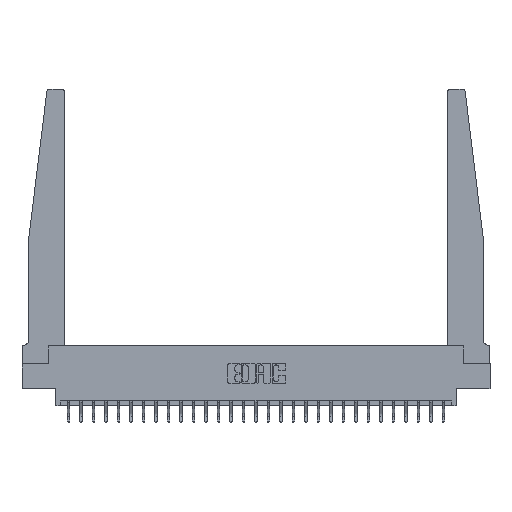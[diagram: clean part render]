
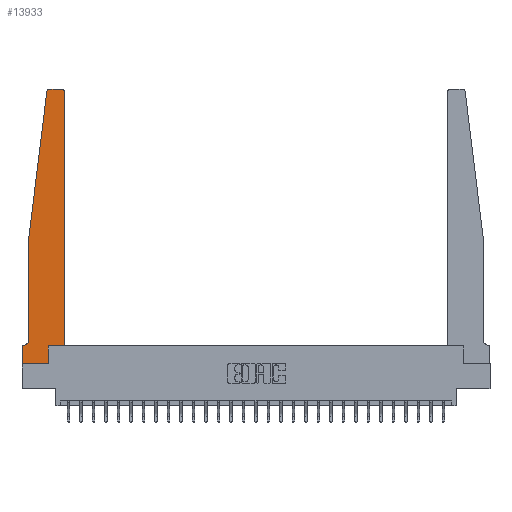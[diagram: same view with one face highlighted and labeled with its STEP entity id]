
A CAD part, top view. The second image highlights one B-rep face of the part: STEP entity #13933.
In plain terms, the highlighted planar face has unit normal (0, 0, 1).
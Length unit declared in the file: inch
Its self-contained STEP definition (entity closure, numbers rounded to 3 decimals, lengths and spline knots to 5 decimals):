
#178 = DIRECTION ( 'NONE',  ( 1., 0., 0. ) ) ;
#185 = DIRECTION ( 'NONE',  ( -1., 0., 0. ) ) ;
#621 = CARTESIAN_POINT ( 'NONE',  ( 0.425, 0.18, 0.37 ) ) ;
#720 = LINE ( 'NONE', #15102, #7549 ) ;
#905 = ORIENTED_EDGE ( 'NONE', *, *, #20341, .T. ) ;
#1428 = VERTEX_POINT ( 'NONE', #9687 ) ;
#1728 = FACE_OUTER_BOUND ( 'NONE', #15883, .T. ) ;
#1777 = VERTEX_POINT ( 'NONE', #15688 ) ;
#1837 = ORIENTED_EDGE ( 'NONE', *, *, #11413, .T. ) ;
#2087 = EDGE_CURVE ( 'NONE', #8320, #10356, #23120, .T. ) ;
#2580 = CARTESIAN_POINT ( 'NONE',  ( 0.015, 0.2375, 0.37 ) ) ;
#3020 = VECTOR ( 'NONE', #24836, 39.37008 ) ;
#3621 = EDGE_CURVE ( 'NONE', #24551, #7787, #3852, .T. ) ;
#3852 = LINE ( 'NONE', #12295, #3020 ) ;
#3930 = CARTESIAN_POINT ( 'NONE',  ( 0., 0.1875, 0.37 ) ) ;
#3963 = LINE ( 'NONE', #621, #8898 ) ;
#4074 = CARTESIAN_POINT ( 'NONE',  ( 0.24675, 2.72367, 0.37 ) ) ;
#4113 = EDGE_CURVE ( 'NONE', #1777, #4133, #22219, .T. ) ;
#4133 = VERTEX_POINT ( 'NONE', #25760 ) ;
#4425 = VERTEX_POINT ( 'NONE', #14247 ) ;
#4759 = AXIS2_PLACEMENT_3D ( 'NONE', #5615, #18304, #26724 ) ;
#5272 = CARTESIAN_POINT ( 'NONE',  ( 0.065, 1.25, 0.37 ) ) ;
#5615 = CARTESIAN_POINT ( 'NONE',  ( 0.395, 2.72, 0.37 ) ) ;
#6169 = CARTESIAN_POINT ( 'NONE',  ( 0.065, 0.1875, 0.37 ) ) ;
#6347 = LINE ( 'NONE', #21106, #18297 ) ;
#6387 = CIRCLE ( 'NONE', #25783, 0.03 ) ;
#6558 = CARTESIAN_POINT ( 'NONE',  ( 0., 0., 0.37 ) ) ;
#6650 = CARTESIAN_POINT ( 'NONE',  ( 0.27653, 2.72, 0.37 ) ) ;
#6946 = EDGE_CURVE ( 'NONE', #16618, #4425, #720, .T. ) ;
#7549 = VECTOR ( 'NONE', #23517, 39.37008 ) ;
#7787 = VERTEX_POINT ( 'NONE', #17882 ) ;
#8205 = AXIS2_PLACEMENT_3D ( 'NONE', #3930, #10163, #20774 ) ;
#8320 = VERTEX_POINT ( 'NONE', #8462 ) ;
#8462 = CARTESIAN_POINT ( 'NONE',  ( 0.395, 2.75, 0.37 ) ) ;
#8898 = VECTOR ( 'NONE', #26035, 39.37008 ) ;
#9370 = CARTESIAN_POINT ( 'NONE',  ( 0.425, 0.18, 0.37 ) ) ;
#9687 = CARTESIAN_POINT ( 'NONE',  ( 0.425, 2.72, 0.37 ) ) ;
#9797 = CARTESIAN_POINT ( 'NONE',  ( 0.27653, 2.75, 0.37 ) ) ;
#9954 = VERTEX_POINT ( 'NONE', #5272 ) ;
#10163 = DIRECTION ( 'NONE',  ( 0., 0., 1. ) ) ;
#10242 = CARTESIAN_POINT ( 'NONE',  ( 0.425, 0.18, 0.37 ) ) ;
#10336 = AXIS2_PLACEMENT_3D ( 'NONE', #2580, #23701, #19147 ) ;
#10356 = VERTEX_POINT ( 'NONE', #9797 ) ;
#11413 = EDGE_CURVE ( 'NONE', #10356, #15060, #6387, .T. ) ;
#11525 = LINE ( 'NONE', #26000, #15228 ) ;
#11565 = VECTOR ( 'NONE', #22717, 39.37008 ) ;
#11840 = EDGE_CURVE ( 'NONE', #15060, #9954, #6347, .T. ) ;
#12295 = CARTESIAN_POINT ( 'NONE',  ( 0., 0., 0.37 ) ) ;
#12315 = ORIENTED_EDGE ( 'NONE', *, *, #3621, .T. ) ;
#12587 = EDGE_CURVE ( 'NONE', #7787, #16618, #12894, .T. ) ;
#12894 = LINE ( 'NONE', #6558, #13046 ) ;
#13046 = VECTOR ( 'NONE', #178, 39.37008 ) ;
#13933 = ADVANCED_FACE ( 'NONE', ( #1728 ), #26854, .T. ) ;
#14226 = LINE ( 'NONE', #10242, #16449 ) ;
#14247 = CARTESIAN_POINT ( 'NONE',  ( 0.2605, 0.18, 0.37 ) ) ;
#14708 = CARTESIAN_POINT ( 'NONE',  ( 0.2605, 0., 0.37 ) ) ;
#15060 = VERTEX_POINT ( 'NONE', #4074 ) ;
#15102 = CARTESIAN_POINT ( 'NONE',  ( 0.2605, 0.18, 0.37 ) ) ;
#15228 = VECTOR ( 'NONE', #19922, 39.37008 ) ;
#15688 = CARTESIAN_POINT ( 'NONE',  ( 0.065, 0.2375, 0.37 ) ) ;
#15883 = EDGE_LOOP ( 'NONE', ( #23024, #1837, #20906, #24942, #17190, #905, #12315, #15890, #24903, #16985, #21485, #25228 ) ) ;
#15890 = ORIENTED_EDGE ( 'NONE', *, *, #12587, .T. ) ;
#16309 = DIRECTION ( 'NONE',  ( 0., 1., 0. ) ) ;
#16449 = VECTOR ( 'NONE', #16309, 39.37008 ) ;
#16460 = EDGE_CURVE ( 'NONE', #1428, #8320, #18410, .T. ) ;
#16618 = VERTEX_POINT ( 'NONE', #14708 ) ;
#16948 = VECTOR ( 'NONE', #185, 39.37008 ) ;
#16985 = ORIENTED_EDGE ( 'NONE', *, *, #20096, .T. ) ;
#17132 = DIRECTION ( 'NONE',  ( 1., 0., 0. ) ) ;
#17190 = ORIENTED_EDGE ( 'NONE', *, *, #4113, .T. ) ;
#17489 = VERTEX_POINT ( 'NONE', #9370 ) ;
#17882 = CARTESIAN_POINT ( 'NONE',  ( 0., 0., 0.37 ) ) ;
#18297 = VECTOR ( 'NONE', #25649, 39.37008 ) ;
#18304 = DIRECTION ( 'NONE',  ( 0., 0., 1. ) ) ;
#18410 = CIRCLE ( 'NONE', #4759, 0.03 ) ;
#18987 = LINE ( 'NONE', #6169, #11565 ) ;
#19147 = DIRECTION ( 'NONE',  ( -1., 0., 0. ) ) ;
#19922 = DIRECTION ( 'NONE',  ( 0., -1., 0. ) ) ;
#20096 = EDGE_CURVE ( 'NONE', #4425, #17489, #3963, .T. ) ;
#20341 = EDGE_CURVE ( 'NONE', #4133, #24551, #18987, .T. ) ;
#20774 = DIRECTION ( 'NONE',  ( 1., 0., 0. ) ) ;
#20906 = ORIENTED_EDGE ( 'NONE', *, *, #11840, .T. ) ;
#21106 = CARTESIAN_POINT ( 'NONE',  ( 0.065, 1.25, 0.37 ) ) ;
#21485 = ORIENTED_EDGE ( 'NONE', *, *, #22492, .T. ) ;
#22219 = CIRCLE ( 'NONE', #10336, 0.05 ) ;
#22492 = EDGE_CURVE ( 'NONE', #17489, #1428, #14226, .T. ) ;
#22717 = DIRECTION ( 'NONE',  ( -1., 0., 0. ) ) ;
#23024 = ORIENTED_EDGE ( 'NONE', *, *, #2087, .T. ) ;
#23120 = LINE ( 'NONE', #24922, #16948 ) ;
#23422 = CARTESIAN_POINT ( 'NONE',  ( 0., 0.1875, 0.37 ) ) ;
#23480 = DIRECTION ( 'NONE',  ( 0., 0., 1. ) ) ;
#23517 = DIRECTION ( 'NONE',  ( 0., 1., 0. ) ) ;
#23701 = DIRECTION ( 'NONE',  ( 0., 0., -1. ) ) ;
#24551 = VERTEX_POINT ( 'NONE', #23422 ) ;
#24836 = DIRECTION ( 'NONE',  ( 0., -1., 0. ) ) ;
#24903 = ORIENTED_EDGE ( 'NONE', *, *, #6946, .T. ) ;
#24922 = CARTESIAN_POINT ( 'NONE',  ( 0.25, 2.75, 0.37 ) ) ;
#24942 = ORIENTED_EDGE ( 'NONE', *, *, #25098, .T. ) ;
#25098 = EDGE_CURVE ( 'NONE', #9954, #1777, #11525, .T. ) ;
#25228 = ORIENTED_EDGE ( 'NONE', *, *, #16460, .T. ) ;
#25649 = DIRECTION ( 'NONE',  ( -0.122, -0.992, 0. ) ) ;
#25760 = CARTESIAN_POINT ( 'NONE',  ( 0.015, 0.1875, 0.37 ) ) ;
#25783 = AXIS2_PLACEMENT_3D ( 'NONE', #6650, #23480, #17132 ) ;
#26000 = CARTESIAN_POINT ( 'NONE',  ( 0.065, 1.25, 0.37 ) ) ;
#26035 = DIRECTION ( 'NONE',  ( 1., 0., 0. ) ) ;
#26724 = DIRECTION ( 'NONE',  ( 1., 0., 0. ) ) ;
#26854 = PLANE ( 'NONE',  #8205 ) ;
